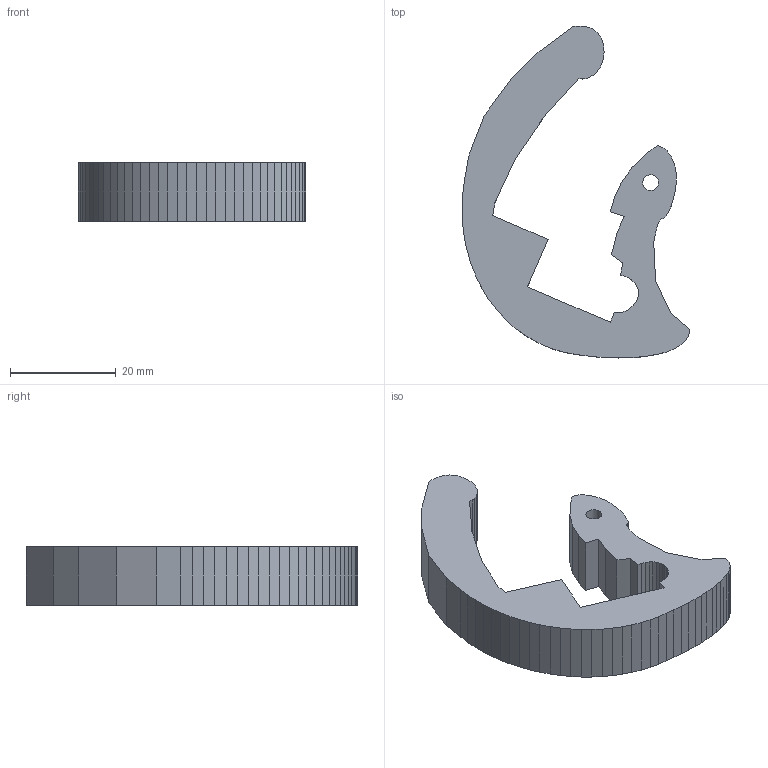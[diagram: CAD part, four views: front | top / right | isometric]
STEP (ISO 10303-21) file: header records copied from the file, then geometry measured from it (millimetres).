
FILE_DESCRIPTION((''),'2;1');
FILE_NAME('trigger.stp','2013-07-10T18:53:09',('mrfr'),(''),'Autodesk Inventor 2013','Autodesk Inventor 2013','');
FILE_SCHEMA(('AUTOMOTIVE_DESIGN { 1 0 10303 214 1 1 1 1 }'));
Length unit declared in the file: millimetre
Products named in the file (1): derringer_mechanika2
Bounding box: 43.13 x 62.82 x 11 mm (x, y, z)
Volume: 11466 mm3; surface area: 5217 mm2
Topology: 1 solids, 1 shells, 139 faces, 411 edges, 274 vertices
Faces by surface type: plane 138, cylinder 1
Full cylindrical faces by diameter (mm): 3 x1
Entity records: 4572 total; most frequent: CARTESIAN_POINT 824, ORIENTED_EDGE 820, DIRECTION 692, EDGE_CURVE 410, VECTOR 408, LINE 408, VERTEX_POINT 274, AXIS2_PLACEMENT_3D 142
